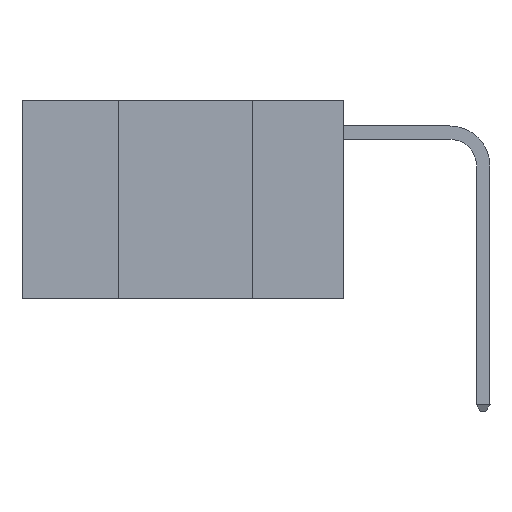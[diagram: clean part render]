
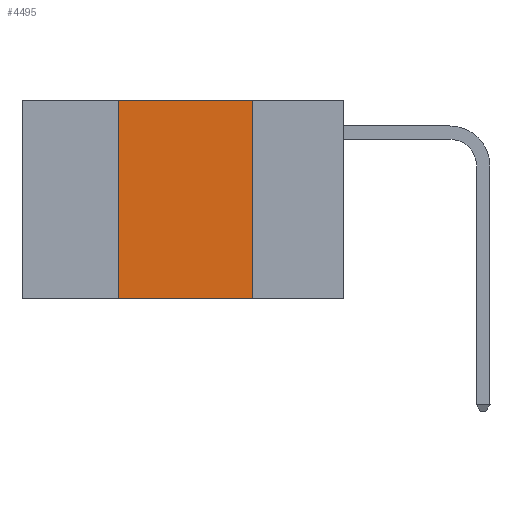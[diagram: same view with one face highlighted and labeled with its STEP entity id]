
A CAD part, left-side view. The second image highlights one B-rep face of the part: STEP entity #4495.
In plain terms, the highlighted planar face has unit normal (-1, 0, 0).
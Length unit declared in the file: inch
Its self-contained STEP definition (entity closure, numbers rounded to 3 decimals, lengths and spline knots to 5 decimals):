
#375 = CARTESIAN_POINT ( 'NONE',  ( 0., 0.6, 0. ) ) ;
#422 = DIRECTION ( 'NONE',  ( 0., 0., -1. ) ) ;
#976 = EDGE_CURVE ( 'NONE', #9396, #5219, #3891, .T. ) ;
#1431 = EDGE_CURVE ( 'NONE', #5219, #5687, #7224, .T. ) ;
#1457 = EDGE_CURVE ( 'NONE', #5247, #9396, #4319, .T. ) ;
#1459 = EDGE_CURVE ( 'NONE', #5247, #5687, #2059, .T. ) ;
#1547 = CARTESIAN_POINT ( 'NONE',  ( 0., 0.42, -0.37 ) ) ;
#1747 = VECTOR ( 'NONE', #11425, 39.37008 ) ;
#2059 = LINE ( 'NONE', #9328, #6690 ) ;
#2390 = VECTOR ( 'NONE', #6551, 39.37008 ) ;
#2639 = CARTESIAN_POINT ( 'NONE',  ( 0., 0.6, 0. ) ) ;
#2834 = ORIENTED_EDGE ( 'NONE', *, *, #976, .F. ) ;
#3081 = DIRECTION ( 'NONE',  ( 0., -1., 0. ) ) ;
#3140 = FACE_OUTER_BOUND ( 'NONE', #9384, .T. ) ;
#3891 = LINE ( 'NONE', #2639, #6041 ) ;
#4077 = DIRECTION ( 'NONE',  ( 0., -1., 0. ) ) ;
#4319 = LINE ( 'NONE', #6076, #1747 ) ;
#4408 = AXIS2_PLACEMENT_3D ( 'NONE', #375, #6068, #422 ) ;
#4495 = ADVANCED_FACE ( 'NONE', ( #3140 ), #5192, .F. ) ;
#5192 = PLANE ( 'NONE',  #4408 ) ;
#5219 = VERTEX_POINT ( 'NONE', #7013 ) ;
#5247 = VERTEX_POINT ( 'NONE', #1547 ) ;
#5687 = VERTEX_POINT ( 'NONE', #9702 ) ;
#6041 = VECTOR ( 'NONE', #4077, 39.37008 ) ;
#6068 = DIRECTION ( 'NONE',  ( 1., 0., 0. ) ) ;
#6076 = CARTESIAN_POINT ( 'NONE',  ( 0., 0.42, 0. ) ) ;
#6339 = CARTESIAN_POINT ( 'NONE',  ( 0., 0.17, 0. ) ) ;
#6551 = DIRECTION ( 'NONE',  ( 0., 0., -1. ) ) ;
#6690 = VECTOR ( 'NONE', #3081, 39.37008 ) ;
#7013 = CARTESIAN_POINT ( 'NONE',  ( 0., 0.17, 0. ) ) ;
#7224 = LINE ( 'NONE', #6339, #2390 ) ;
#7266 = ORIENTED_EDGE ( 'NONE', *, *, #1459, .T. ) ;
#7376 = ORIENTED_EDGE ( 'NONE', *, *, #1457, .F. ) ;
#8063 = ORIENTED_EDGE ( 'NONE', *, *, #1431, .F. ) ;
#9328 = CARTESIAN_POINT ( 'NONE',  ( 0., 0.6, -0.37 ) ) ;
#9384 = EDGE_LOOP ( 'NONE', ( #8063, #2834, #7376, #7266 ) ) ;
#9396 = VERTEX_POINT ( 'NONE', #9914 ) ;
#9702 = CARTESIAN_POINT ( 'NONE',  ( 0., 0.17, -0.37 ) ) ;
#9914 = CARTESIAN_POINT ( 'NONE',  ( 0., 0.42, 0. ) ) ;
#11425 = DIRECTION ( 'NONE',  ( 0., 0., 1. ) ) ;
